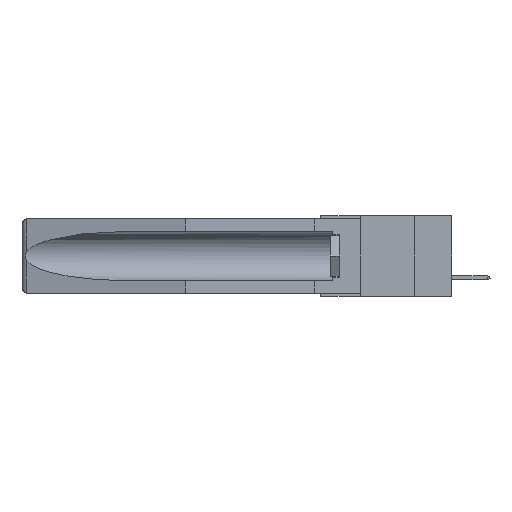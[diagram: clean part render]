
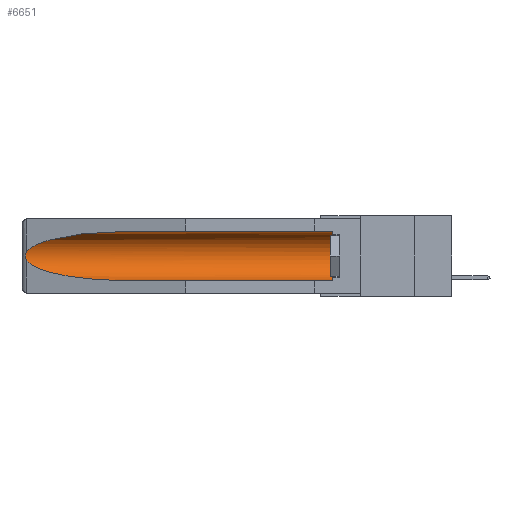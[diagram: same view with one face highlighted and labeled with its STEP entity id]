
A CAD part, left-side view. The second image highlights one B-rep face of the part: STEP entity #6651.
In plain terms, the highlighted cylindrical face has radius 2.857 mm (diameter 5.715 mm), a partial arc.
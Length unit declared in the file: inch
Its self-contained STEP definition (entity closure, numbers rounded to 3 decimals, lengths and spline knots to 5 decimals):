
#114 = CARTESIAN_POINT ( 'NONE',  ( 0.155, -0.30754, -0.1715 ) ) ;
#461 = ORIENTED_EDGE ( 'NONE', *, *, #16210, .T. ) ;
#1164 = VERTEX_POINT ( 'NONE', #8871 ) ;
#1194 = CARTESIAN_POINT ( 'NONE',  ( 0.155, 1.07973, -0.284 ) ) ;
#2988 = ORIENTED_EDGE ( 'NONE', *, *, #10881, .T. ) ;
#3165 = EDGE_CURVE ( 'NONE', #22612, #24288, #6095, .T. ) ;
#3427 = AXIS2_PLACEMENT_3D ( 'NONE', #114, #15282, #13459 ) ;
#4929 = CARTESIAN_POINT ( 'NONE',  ( 0.155, 1.07973, -0.284 ) ) ;
#5349 = CYLINDRICAL_SURFACE ( 'NONE', #3427, 0.1125 ) ;
#5431 = EDGE_LOOP ( 'NONE', ( #20665, #16160, #19642, #15164, #461, #2988 ) ) ;
#6095 = LINE ( 'NONE', #22246, #16567 ) ;
#6419 = CARTESIAN_POINT ( 'NONE',  ( 0.26597, 1.52961, -0.15275 ) ) ;
#6502 = CARTESIAN_POINT ( 'NONE',  ( 0.2673, 1.53269, -0.17917 ) ) ;
#6584 = CARTESIAN_POINT ( 'NONE',  ( 0.26654, 1.53092, -0.15636 ) ) ;
#6651 = ADVANCED_FACE ( 'NONE', ( #20818 ), #5349, .F. ) ;
#7202 = EDGE_CURVE ( 'NONE', #17719, #24288, #10949, .T. ) ;
#7308 = CARTESIAN_POINT ( 'NONE',  ( 0.155, -0.30754, -0.059 ) ) ;
#7566 = DIRECTION ( 'NONE',  ( 0., -1., 0. ) ) ;
#8299 = VECTOR ( 'NONE', #22090, 39.37008 ) ;
#8405 = EDGE_CURVE ( 'NONE', #9081, #1164, #13991, .T. ) ;
#8453 = CARTESIAN_POINT ( 'NONE',  ( 0.26537, 1.52718, -0.19328 ) ) ;
#8846 = AXIS2_PLACEMENT_3D ( 'NONE', #22897, #7566, #15141 ) ;
#8871 = CARTESIAN_POINT ( 'NONE',  ( 0.26537, 1.52718, -0.14972 ) ) ;
#9081 = VERTEX_POINT ( 'NONE', #14125 ) ;
#10446 = CARTESIAN_POINT ( 'NONE',  ( 0.26655, 1.53094, -0.18657 ) ) ;
#10528 = CARTESIAN_POINT ( 'NONE',  ( 0.26597, 1.5296, -0.19026 ) ) ;
#10881 = EDGE_CURVE ( 'NONE', #11420, #9081, #22561, .T. ) ;
#10949 =( BOUNDED_CURVE ( )  B_SPLINE_CURVE ( 3, ( #12645, #20056, #18092, #4929 ),
 .UNSPECIFIED., .F., .F. ) 
 B_SPLINE_CURVE_WITH_KNOTS ( ( 4, 4 ),
 ( 0.1948, 1.5708 ),
 .UNSPECIFIED. ) 
 CURVE ( )  GEOMETRIC_REPRESENTATION_ITEM ( )  RATIONAL_B_SPLINE_CURVE ( ( 1., 0.848, 0.848, 1. ) ) 
 REPRESENTATION_ITEM ( '' )  );
#11420 = VERTEX_POINT ( 'NONE', #17182 ) ;
#12645 = CARTESIAN_POINT ( 'NONE',  ( 0.26537, 1.52718, -0.19328 ) ) ;
#13459 = DIRECTION ( 'NONE',  ( 0., 0., 1. ) ) ;
#13991 =( BOUNDED_CURVE ( )  B_SPLINE_CURVE ( 3, ( #18918, #16840, #22628, #17161 ),
 .UNSPECIFIED., .F., .F. ) 
 B_SPLINE_CURVE_WITH_KNOTS ( ( 4, 4 ),
 ( 4.71239, 6.08839 ),
 .UNSPECIFIED. ) 
 CURVE ( )  GEOMETRIC_REPRESENTATION_ITEM ( )  RATIONAL_B_SPLINE_CURVE ( ( 1., 0.848, 0.848, 1. ) ) 
 REPRESENTATION_ITEM ( '' )  );
#14125 = CARTESIAN_POINT ( 'NONE',  ( 0.155, 1.07973, -0.059 ) ) ;
#14209 = CARTESIAN_POINT ( 'NONE',  ( 0.2675, 1.53308, -0.17534 ) ) ;
#15141 = DIRECTION ( 'NONE',  ( 0., 0., 1. ) ) ;
#15164 = ORIENTED_EDGE ( 'NONE', *, *, #3165, .F. ) ;
#15282 = DIRECTION ( 'NONE',  ( 0., 1., 0. ) ) ;
#15452 = CIRCLE ( 'NONE', #8846, 0.1125 ) ;
#15632 = CARTESIAN_POINT ( 'NONE',  ( 0.155, 0.126, -0.284 ) ) ;
#16160 = ORIENTED_EDGE ( 'NONE', *, *, #19880, .T. ) ;
#16210 = EDGE_CURVE ( 'NONE', #22612, #11420, #15452, .T. ) ;
#16567 = VECTOR ( 'NONE', #23893, 39.37008 ) ;
#16840 = CARTESIAN_POINT ( 'NONE',  ( 0.21114, 1.30732, -0.059 ) ) ;
#17161 = CARTESIAN_POINT ( 'NONE',  ( 0.26537, 1.52718, -0.14972 ) ) ;
#17182 = CARTESIAN_POINT ( 'NONE',  ( 0.155, 0.126, -0.059 ) ) ;
#17455 = CARTESIAN_POINT ( 'NONE',  ( 0.26537, 1.52718, -0.19328 ) ) ;
#17719 = VERTEX_POINT ( 'NONE', #17455 ) ;
#18092 = CARTESIAN_POINT ( 'NONE',  ( 0.21114, 1.30732, -0.284 ) ) ;
#18918 = CARTESIAN_POINT ( 'NONE',  ( 0.155, 1.07973, -0.059 ) ) ;
#19482 = CARTESIAN_POINT ( 'NONE',  ( 0.26537, 1.52718, -0.14972 ) ) ;
#19642 = ORIENTED_EDGE ( 'NONE', *, *, #7202, .T. ) ;
#19880 = EDGE_CURVE ( 'NONE', #1164, #17719, #24171, .T. ) ;
#19885 = CARTESIAN_POINT ( 'NONE',  ( 0.2675, 1.53308, -0.16763 ) ) ;
#20056 = CARTESIAN_POINT ( 'NONE',  ( 0.25451, 1.48313, -0.24835 ) ) ;
#20665 = ORIENTED_EDGE ( 'NONE', *, *, #8405, .T. ) ;
#20818 = FACE_OUTER_BOUND ( 'NONE', #5431, .T. ) ;
#21803 = CARTESIAN_POINT ( 'NONE',  ( 0.2673, 1.5327, -0.16383 ) ) ;
#22090 = DIRECTION ( 'NONE',  ( 0., 1., 0. ) ) ;
#22246 = CARTESIAN_POINT ( 'NONE',  ( 0.155, -0.30754, -0.284 ) ) ;
#22561 = LINE ( 'NONE', #7308, #8299 ) ;
#22612 = VERTEX_POINT ( 'NONE', #15632 ) ;
#22628 = CARTESIAN_POINT ( 'NONE',  ( 0.25451, 1.48313, -0.09465 ) ) ;
#22897 = CARTESIAN_POINT ( 'NONE',  ( 0.155, 0.126, -0.1715 ) ) ;
#23893 = DIRECTION ( 'NONE',  ( 0., 1., 0. ) ) ;
#24171 = B_SPLINE_CURVE_WITH_KNOTS ( 'NONE', 3,
 ( #19482, #6419, #6584, #21803, #19885, #14209, #6502, #10446, #10528, #8453 ),
 .UNSPECIFIED., .F., .F.,
 ( 4, 2, 2, 2, 4 ),
 ( 0., 0.00029, 0.00058, 0.00087, 0.00117 ),
 .UNSPECIFIED. ) ;
#24288 = VERTEX_POINT ( 'NONE', #1194 ) ;
